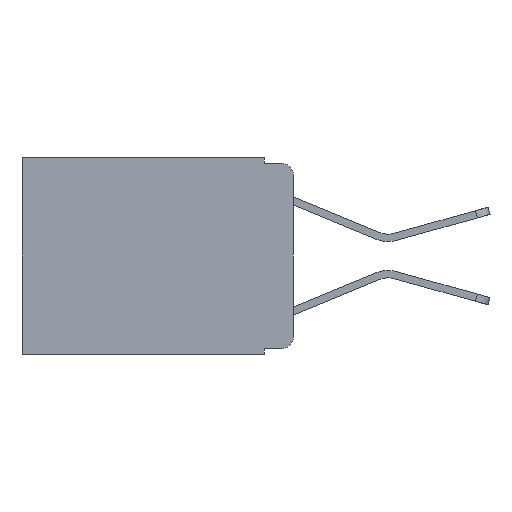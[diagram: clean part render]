
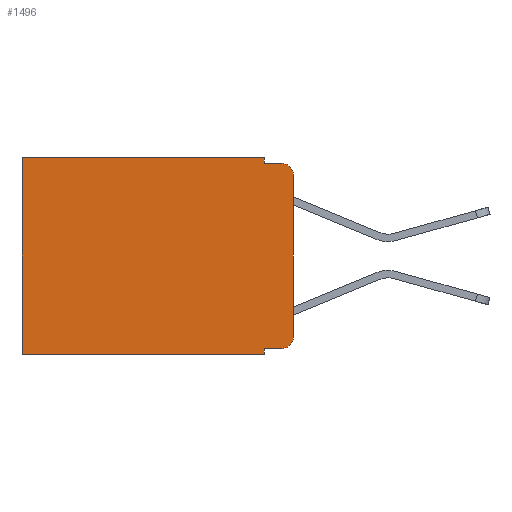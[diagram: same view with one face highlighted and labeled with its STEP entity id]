
A CAD part, left-side view. The second image highlights one B-rep face of the part: STEP entity #1496.
In plain terms, the highlighted planar face has unit normal (-1, 0, 0).
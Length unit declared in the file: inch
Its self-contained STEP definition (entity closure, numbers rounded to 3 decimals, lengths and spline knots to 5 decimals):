
#91 = CARTESIAN_POINT ( 'NONE',  ( 0.298, 0.051, -0.343 ) ) ;
#104 = DIRECTION ( 'NONE',  ( 0., 0., -1. ) ) ;
#106 = LINE ( 'NONE', #9806, #9434 ) ;
#141 = VERTEX_POINT ( 'NONE', #8339 ) ;
#144 = VERTEX_POINT ( 'NONE', #10451 ) ;
#155 = VECTOR ( 'NONE', #4286, 39.37008 ) ;
#334 = VERTEX_POINT ( 'NONE', #6591 ) ;
#483 = LINE ( 'NONE', #8344, #155 ) ;
#494 = ORIENTED_EDGE ( 'NONE', *, *, #8311, .F. ) ;
#802 = VERTEX_POINT ( 'NONE', #4643 ) ;
#809 = CARTESIAN_POINT ( 'NONE',  ( 0.298, 0.02, -0.333 ) ) ;
#1103 = VECTOR ( 'NONE', #9096, 39.37008 ) ;
#1193 = VERTEX_POINT ( 'NONE', #2665 ) ;
#1280 = VERTEX_POINT ( 'NONE', #91 ) ;
#1358 = DIRECTION ( 'NONE',  ( 0., -1., 0. ) ) ;
#1400 = CARTESIAN_POINT ( 'NONE',  ( 0.298, 0.473, 0. ) ) ;
#1413 = AXIS2_PLACEMENT_3D ( 'NONE', #5142, #9823, #6804 ) ;
#1496 = ADVANCED_FACE ( 'NONE', ( #4940 ), #1599, .F. ) ;
#1599 = PLANE ( 'NONE',  #1413 ) ;
#1885 = AXIS2_PLACEMENT_3D ( 'NONE', #2504, #8363, #3439 ) ;
#1939 = VERTEX_POINT ( 'NONE', #1400 ) ;
#2341 = EDGE_CURVE ( 'NONE', #802, #1939, #4977, .T. ) ;
#2396 = ORIENTED_EDGE ( 'NONE', *, *, #2470, .F. ) ;
#2470 = EDGE_CURVE ( 'NONE', #144, #1193, #8010, .T. ) ;
#2504 = CARTESIAN_POINT ( 'NONE',  ( 0.298, 0.02, -0.03 ) ) ;
#2601 = VECTOR ( 'NONE', #3452, 39.37008 ) ;
#2665 = CARTESIAN_POINT ( 'NONE',  ( 0.298, 0., -0.313 ) ) ;
#2693 = ORIENTED_EDGE ( 'NONE', *, *, #9785, .F. ) ;
#2824 = CARTESIAN_POINT ( 'NONE',  ( 0.298, 0.051, 0. ) ) ;
#2986 = ORIENTED_EDGE ( 'NONE', *, *, #2341, .T. ) ;
#3082 = CARTESIAN_POINT ( 'NONE',  ( 0.298, 0.051, -0.333 ) ) ;
#3142 = CARTESIAN_POINT ( 'NONE',  ( 0.298, 0.02, -0.313 ) ) ;
#3192 = LINE ( 'NONE', #2824, #9185 ) ;
#3275 = ORIENTED_EDGE ( 'NONE', *, *, #7344, .F. ) ;
#3439 = DIRECTION ( 'NONE',  ( 0., 0., -1. ) ) ;
#3452 = DIRECTION ( 'NONE',  ( 0., 1., 0. ) ) ;
#3472 = AXIS2_PLACEMENT_3D ( 'NONE', #3142, #8873, #4022 ) ;
#4022 = DIRECTION ( 'NONE',  ( 0., 0., -1. ) ) ;
#4286 = DIRECTION ( 'NONE',  ( 0., -1., 0. ) ) ;
#4630 = VERTEX_POINT ( 'NONE', #3082 ) ;
#4643 = CARTESIAN_POINT ( 'NONE',  ( 0.298, 0.051, 0. ) ) ;
#4940 = FACE_OUTER_BOUND ( 'NONE', #9121, .T. ) ;
#4977 = LINE ( 'NONE', #5216, #2601 ) ;
#5142 = CARTESIAN_POINT ( 'NONE',  ( 0.298, 0., 0. ) ) ;
#5216 = CARTESIAN_POINT ( 'NONE',  ( 0.298, 0., 0. ) ) ;
#5239 = CARTESIAN_POINT ( 'NONE',  ( 0.298, 0.02, -0.01 ) ) ;
#5358 = ORIENTED_EDGE ( 'NONE', *, *, #7834, .T. ) ;
#5452 = CIRCLE ( 'NONE', #3472, 0.02 ) ;
#5708 = EDGE_CURVE ( 'NONE', #9359, #1193, #5452, .T. ) ;
#5915 = LINE ( 'NONE', #8173, #7532 ) ;
#5942 = VECTOR ( 'NONE', #104, 39.37008 ) ;
#6060 = CARTESIAN_POINT ( 'NONE',  ( 0.298, 0.473, 0. ) ) ;
#6110 = VECTOR ( 'NONE', #1358, 39.37008 ) ;
#6296 = EDGE_CURVE ( 'NONE', #4630, #9359, #6392, .T. ) ;
#6392 = LINE ( 'NONE', #6719, #6110 ) ;
#6425 = EDGE_CURVE ( 'NONE', #1280, #141, #106, .T. ) ;
#6591 = CARTESIAN_POINT ( 'NONE',  ( 0.298, 0.051, -0.01 ) ) ;
#6719 = CARTESIAN_POINT ( 'NONE',  ( 0.298, 0.051, -0.333 ) ) ;
#6731 = CARTESIAN_POINT ( 'NONE',  ( 0.298, 0., 0. ) ) ;
#6804 = DIRECTION ( 'NONE',  ( 0., 0., -1. ) ) ;
#7134 = DIRECTION ( 'NONE',  ( 0., 0., -1. ) ) ;
#7344 = EDGE_CURVE ( 'NONE', #4630, #1280, #3192, .T. ) ;
#7532 = VECTOR ( 'NONE', #8889, 39.37008 ) ;
#7834 = EDGE_CURVE ( 'NONE', #1939, #141, #9936, .T. ) ;
#7979 = ORIENTED_EDGE ( 'NONE', *, *, #5708, .T. ) ;
#8010 = LINE ( 'NONE', #6731, #5942 ) ;
#8173 = CARTESIAN_POINT ( 'NONE',  ( 0.298, 0.051, 0. ) ) ;
#8311 = EDGE_CURVE ( 'NONE', #802, #334, #5915, .T. ) ;
#8339 = CARTESIAN_POINT ( 'NONE',  ( 0.298, 0.473, -0.343 ) ) ;
#8344 = CARTESIAN_POINT ( 'NONE',  ( 0.298, 0.051, -0.01 ) ) ;
#8363 = DIRECTION ( 'NONE',  ( -1., 0., 0. ) ) ;
#8873 = DIRECTION ( 'NONE',  ( -1., 0., 0. ) ) ;
#8889 = DIRECTION ( 'NONE',  ( 0., 0., -1. ) ) ;
#9023 = ORIENTED_EDGE ( 'NONE', *, *, #10278, .T. ) ;
#9096 = DIRECTION ( 'NONE',  ( 0., 0., -1. ) ) ;
#9121 = EDGE_LOOP ( 'NONE', ( #2396, #9023, #2693, #494, #2986, #5358, #9480, #3275, #9698, #7979 ) ) ;
#9185 = VECTOR ( 'NONE', #7134, 39.37008 ) ;
#9287 = VERTEX_POINT ( 'NONE', #5239 ) ;
#9359 = VERTEX_POINT ( 'NONE', #809 ) ;
#9434 = VECTOR ( 'NONE', #9832, 39.37008 ) ;
#9480 = ORIENTED_EDGE ( 'NONE', *, *, #6425, .F. ) ;
#9698 = ORIENTED_EDGE ( 'NONE', *, *, #6296, .T. ) ;
#9785 = EDGE_CURVE ( 'NONE', #334, #9287, #483, .T. ) ;
#9806 = CARTESIAN_POINT ( 'NONE',  ( 0.298, 0., -0.343 ) ) ;
#9823 = DIRECTION ( 'NONE',  ( 1., 0., 0. ) ) ;
#9832 = DIRECTION ( 'NONE',  ( 0., 1., 0. ) ) ;
#9936 = LINE ( 'NONE', #6060, #1103 ) ;
#10278 = EDGE_CURVE ( 'NONE', #144, #9287, #10711, .T. ) ;
#10451 = CARTESIAN_POINT ( 'NONE',  ( 0.298, 0., -0.03 ) ) ;
#10711 = CIRCLE ( 'NONE', #1885, 0.02 ) ;
